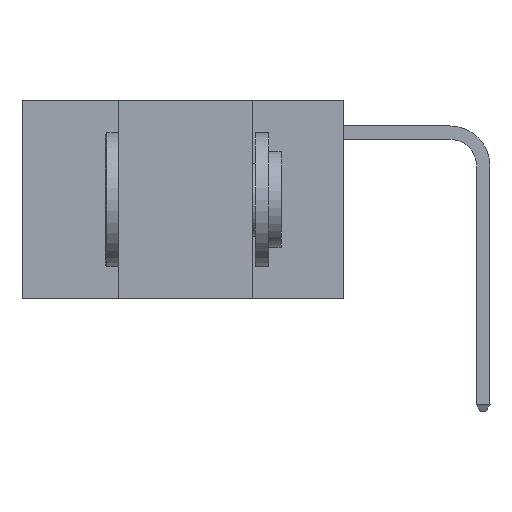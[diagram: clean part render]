
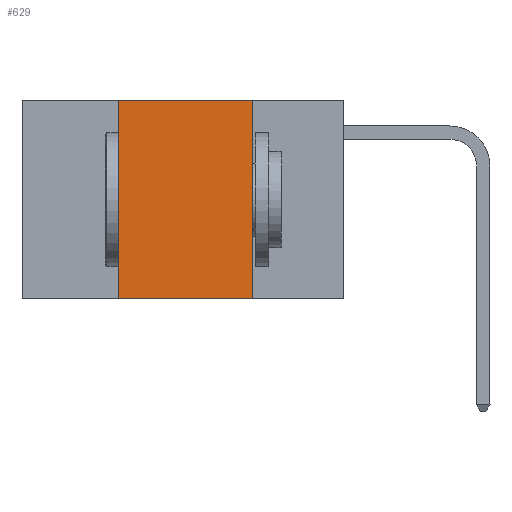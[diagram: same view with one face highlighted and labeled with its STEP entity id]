
A CAD part, left-side view. The second image highlights one B-rep face of the part: STEP entity #629.
In plain terms, the highlighted planar face has unit normal (-1, 0, 0).
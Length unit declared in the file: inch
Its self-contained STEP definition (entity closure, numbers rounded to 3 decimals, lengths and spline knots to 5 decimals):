
#563 = EDGE_LOOP ( 'NONE', ( #17912, #18460, #4778, #9596 ) ) ;
#629 = ADVANCED_FACE ( 'NONE', ( #1499 ), #13477, .F. ) ;
#1499 = FACE_OUTER_BOUND ( 'NONE', #563, .T. ) ;
#2691 = EDGE_CURVE ( 'NONE', #3292, #8872, #9974, .T. ) ;
#3292 = VERTEX_POINT ( 'NONE', #13534 ) ;
#3943 = CARTESIAN_POINT ( 'NONE',  ( 0., 0.17, -0.37 ) ) ;
#4260 = CARTESIAN_POINT ( 'NONE',  ( 0., 0.6, -0.37 ) ) ;
#4744 = CARTESIAN_POINT ( 'NONE',  ( 0., 0.17, 0. ) ) ;
#4778 = ORIENTED_EDGE ( 'NONE', *, *, #14412, .F. ) ;
#5839 = VERTEX_POINT ( 'NONE', #19563 ) ;
#5859 = VECTOR ( 'NONE', #6829, 39.37008 ) ;
#6829 = DIRECTION ( 'NONE',  ( 0., -1., 0. ) ) ;
#8418 = VERTEX_POINT ( 'NONE', #17172 ) ;
#8872 = VERTEX_POINT ( 'NONE', #3943 ) ;
#9288 = DIRECTION ( 'NONE',  ( 0., 0., 1. ) ) ;
#9596 = ORIENTED_EDGE ( 'NONE', *, *, #13512, .T. ) ;
#9637 = DIRECTION ( 'NONE',  ( 0., -1., 0. ) ) ;
#9974 = LINE ( 'NONE', #4744, #18829 ) ;
#9988 = EDGE_CURVE ( 'NONE', #5839, #3292, #20578, .T. ) ;
#12096 = AXIS2_PLACEMENT_3D ( 'NONE', #14456, #13447, #13368 ) ;
#13307 = LINE ( 'NONE', #4260, #17994 ) ;
#13368 = DIRECTION ( 'NONE',  ( 0., 0., -1. ) ) ;
#13447 = DIRECTION ( 'NONE',  ( 1., 0., 0. ) ) ;
#13477 = PLANE ( 'NONE',  #12096 ) ;
#13512 = EDGE_CURVE ( 'NONE', #8418, #8872, #13307, .T. ) ;
#13534 = CARTESIAN_POINT ( 'NONE',  ( 0., 0.17, 0. ) ) ;
#13549 = LINE ( 'NONE', #21620, #17668 ) ;
#14412 = EDGE_CURVE ( 'NONE', #8418, #5839, #13549, .T. ) ;
#14456 = CARTESIAN_POINT ( 'NONE',  ( 0., 0.6, 0. ) ) ;
#17172 = CARTESIAN_POINT ( 'NONE',  ( 0., 0.42, -0.37 ) ) ;
#17253 = DIRECTION ( 'NONE',  ( 0., 0., -1. ) ) ;
#17668 = VECTOR ( 'NONE', #9288, 39.37008 ) ;
#17912 = ORIENTED_EDGE ( 'NONE', *, *, #2691, .F. ) ;
#17994 = VECTOR ( 'NONE', #9637, 39.37008 ) ;
#18460 = ORIENTED_EDGE ( 'NONE', *, *, #9988, .F. ) ;
#18829 = VECTOR ( 'NONE', #17253, 39.37008 ) ;
#19563 = CARTESIAN_POINT ( 'NONE',  ( 0., 0.42, 0. ) ) ;
#20578 = LINE ( 'NONE', #21006, #5859 ) ;
#21006 = CARTESIAN_POINT ( 'NONE',  ( 0., 0.6, 0. ) ) ;
#21620 = CARTESIAN_POINT ( 'NONE',  ( 0., 0.42, 0. ) ) ;
